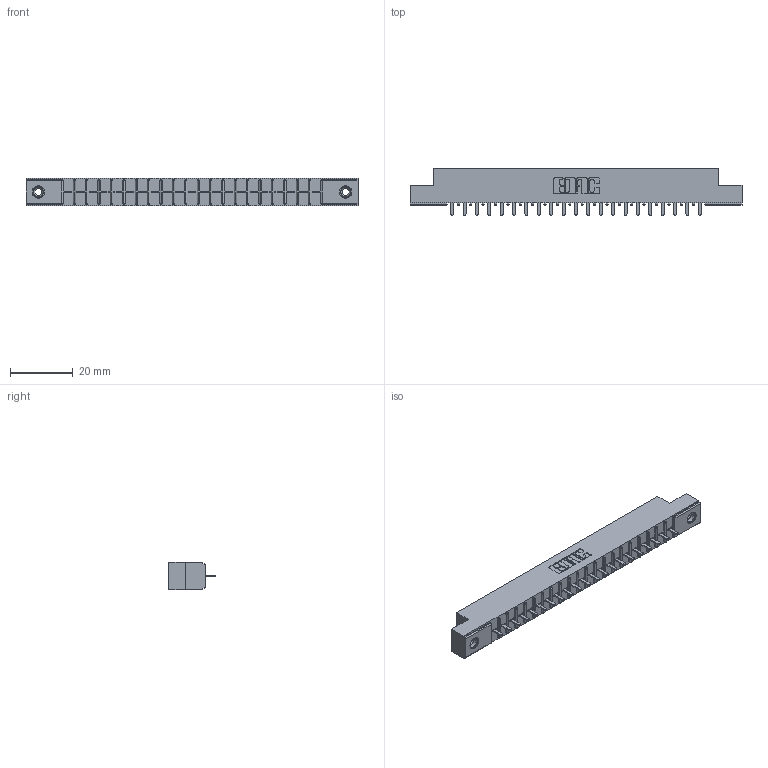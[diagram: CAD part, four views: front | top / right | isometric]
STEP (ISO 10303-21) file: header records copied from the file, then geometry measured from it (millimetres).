
FILE_DESCRIPTION (( 'STEP AP203' ), '1' );
FILE_NAME ('316-021-521-108.STEP', '2018-07-31T01:48:23', ( '' ), ( '' ), 'SwSTEP 2.0', 'SolidWorks 2016', '' );
FILE_SCHEMA (( 'CONFIG_CONTROL_DESIGN' ));
Length unit declared in the file: inch
Products named in the file (4): 306 Part_.156 Dia; 306-290-001_121; 345-250-001_345-250-003-102; 316-021-521-108
Assembly tree (24 placements, depth 2):
  316-021-521-108
    306 Part_.156 Dia
    306-290-001_121  x21
    345-250-001_345-250-003-102  x2
Bounding box: 106.22 x 14.88 x 8.71 mm (x, y, z)
Volume: 7230.8 mm3; surface area: 10528.8 mm2
Topology: 24 solids, 24 shells, 1646 faces, 4589 edges, 2938 vertices
Faces by surface type: plane 1087, cylinder 459, sphere 84, cone 12, torus 4
Entity records: 23445 total; most frequent: CARTESIAN_POINT 3913, ORIENTED_EDGE 3870, DIRECTION 3869, EDGE_CURVE 1935, LINE 1501, VECTOR 1501, VERTEX_POINT 1228, AXIS2_PLACEMENT_3D 1184
